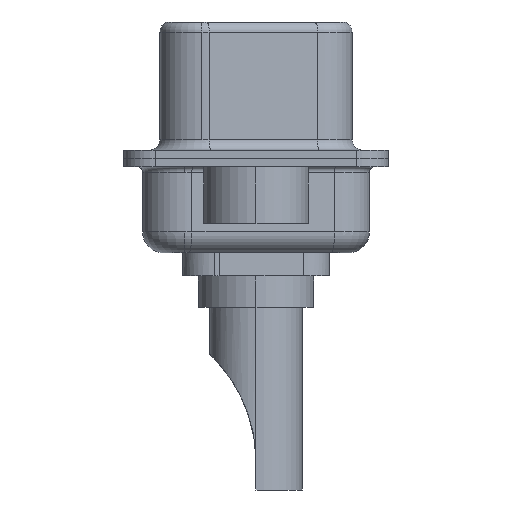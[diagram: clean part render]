
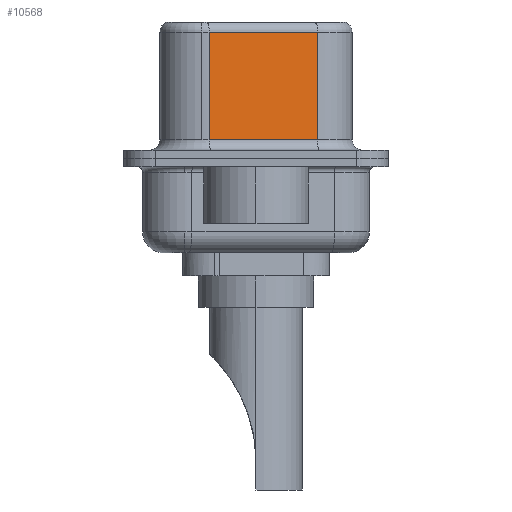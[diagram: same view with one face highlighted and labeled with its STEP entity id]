
A CAD part, left-side view. The second image highlights one B-rep face of the part: STEP entity #10568.
In plain terms, the highlighted planar face has unit normal (-0.985, -0.174, 0).
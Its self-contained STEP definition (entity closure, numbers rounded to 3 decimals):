
#242 = ORIENTED_EDGE ( 'NONE', *, *, #17107, .F. ) ;
#259 = ORIENTED_EDGE ( 'NONE', *, *, #16091, .T. ) ;
#1129 = DIRECTION ( 'NONE',  ( -0.174, 0.985, 0. ) ) ;
#1636 = DIRECTION ( 'NONE',  ( -0.174, 0.985, 0. ) ) ;
#1905 = VERTEX_POINT ( 'NONE', #5524 ) ;
#2253 = LINE ( 'NONE', #9960, #10019 ) ;
#2429 = VERTEX_POINT ( 'NONE', #14109 ) ;
#3754 = CARTESIAN_POINT ( 'NONE',  ( 4.585, -2.927, 0.9 ) ) ;
#4746 = VERTEX_POINT ( 'NONE', #18453 ) ;
#5524 = CARTESIAN_POINT ( 'NONE',  ( 4.585, -2.927, 6.02 ) ) ;
#5540 = CARTESIAN_POINT ( 'NONE',  ( 3.675, 2.233, 6.52 ) ) ;
#7208 = DIRECTION ( 'NONE',  ( 0., 0., -1. ) ) ;
#7504 = EDGE_CURVE ( 'NONE', #13723, #2429, #8042, .T. ) ;
#7524 = VECTOR ( 'NONE', #7208, 1000. ) ;
#8042 = LINE ( 'NONE', #5540, #7524 ) ;
#9888 = DIRECTION ( 'NONE',  ( 0., 0., -1. ) ) ;
#9960 = CARTESIAN_POINT ( 'NONE',  ( 4.585, -2.927, 6.52 ) ) ;
#10019 = VECTOR ( 'NONE', #9888, 1000. ) ;
#10415 = ORIENTED_EDGE ( 'NONE', *, *, #11331, .T. ) ;
#10568 = ADVANCED_FACE ( 'NONE', ( #21287 ), #20891, .F. ) ;
#10833 = VECTOR ( 'NONE', #1636, 1000. ) ;
#11062 = DIRECTION ( 'NONE',  ( 0.985, 0.174, 0. ) ) ;
#11331 = EDGE_CURVE ( 'NONE', #2429, #4746, #15840, .T. ) ;
#11337 = LINE ( 'NONE', #21392, #10833 ) ;
#13265 = EDGE_LOOP ( 'NONE', ( #242, #259, #18834, #10415 ) ) ;
#13723 = VERTEX_POINT ( 'NONE', #19524 ) ;
#14109 = CARTESIAN_POINT ( 'NONE',  ( 3.675, 2.233, 0.9 ) ) ;
#14824 = VECTOR ( 'NONE', #15241, 1000. ) ;
#15241 = DIRECTION ( 'NONE',  ( 0.174, -0.985, 0. ) ) ;
#15840 = LINE ( 'NONE', #3754, #14824 ) ;
#16091 = EDGE_CURVE ( 'NONE', #1905, #13723, #11337, .T. ) ;
#17107 = EDGE_CURVE ( 'NONE', #1905, #4746, #2253, .T. ) ;
#18453 = CARTESIAN_POINT ( 'NONE',  ( 4.585, -2.927, 0.9 ) ) ;
#18834 = ORIENTED_EDGE ( 'NONE', *, *, #7504, .T. ) ;
#19218 = CARTESIAN_POINT ( 'NONE',  ( 4.585, -2.927, 6.52 ) ) ;
#19524 = CARTESIAN_POINT ( 'NONE',  ( 3.675, 2.233, 6.02 ) ) ;
#20532 = AXIS2_PLACEMENT_3D ( 'NONE', #19218, #11062, #1129 ) ;
#20891 = PLANE ( 'NONE',  #20532 ) ;
#21287 = FACE_OUTER_BOUND ( 'NONE', #13265, .T. ) ;
#21392 = CARTESIAN_POINT ( 'NONE',  ( 4.585, -2.927, 6.02 ) ) ;
